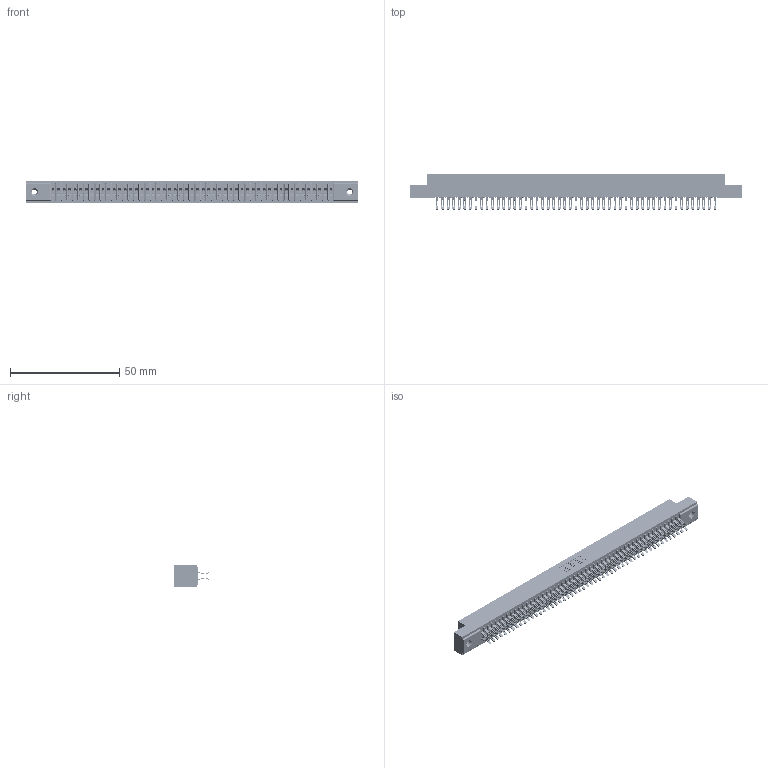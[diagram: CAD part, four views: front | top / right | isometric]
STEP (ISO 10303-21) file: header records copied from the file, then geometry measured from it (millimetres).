
FILE_DESCRIPTION (( 'STEP AP203' ), '1' );
FILE_NAME ('391-102-555-208.STEP', '2018-08-09T20:02:23', ( '' ), ( '' ), 'SwSTEP 2.0', 'SolidWorks 2016', '' );
FILE_SCHEMA (( 'CONFIG_CONTROL_DESIGN' ));
Length unit declared in the file: inch
Products named in the file (4): 391-102-555-208; 341 Part_.156 (3.96) Dia Mounting Holes; 341-292-001_341-292-155; 345-250-001_345-250-003-102
Assembly tree (105 placements, depth 2):
  391-102-555-208
    341 Part_.156 (3.96) Dia Mounting Holes
    341-292-001_341-292-155  x102
    345-250-001_345-250-003-102  x2
Bounding box: 151.76 x 16.31 x 10.16 mm (x, y, z)
Volume: 11338.1 mm3; surface area: 21261.9 mm2
Topology: 105 solids, 105 shells, 8132 faces, 24269 edges, 15794 vertices
Faces by surface type: plane 4384, cylinder 3528, sphere 104, torus 104, cone 12
Entity records: 62177 total; most frequent: CARTESIAN_POINT 10334, ORIENTED_EDGE 10254, DIRECTION 10023, EDGE_CURVE 5127, LINE 4133, VECTOR 4133, VERTEX_POINT 3240, AXIS2_PLACEMENT_3D 2945
